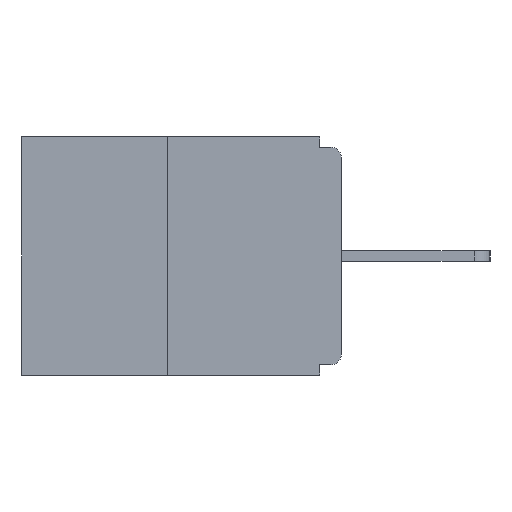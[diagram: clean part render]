
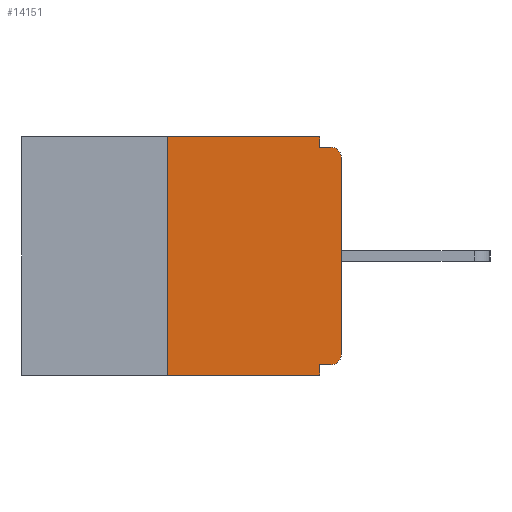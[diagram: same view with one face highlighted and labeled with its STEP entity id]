
A CAD part, left-side view. The second image highlights one B-rep face of the part: STEP entity #14151.
In plain terms, the highlighted planar face has unit normal (-1, 0, 0).
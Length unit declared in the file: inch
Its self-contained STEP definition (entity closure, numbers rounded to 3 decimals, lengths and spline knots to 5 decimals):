
#359 = VECTOR ( 'NONE', #7062, 39.37008 ) ;
#1234 = VECTOR ( 'NONE', #3320, 39.37008 ) ;
#2044 = EDGE_LOOP ( 'NONE', ( #13302, #2677, #19557, #24376, #18803, #3095, #15325, #21957, #6473, #6462 ) ) ;
#2048 = CARTESIAN_POINT ( 'NONE',  ( 0., 0.031, -0.015 ) ) ;
#2384 = VERTEX_POINT ( 'NONE', #6562 ) ;
#2677 = ORIENTED_EDGE ( 'NONE', *, *, #5023, .F. ) ;
#2897 = VERTEX_POINT ( 'NONE', #3703 ) ;
#2973 = AXIS2_PLACEMENT_3D ( 'NONE', #21497, #9699, #23426 ) ;
#3095 = ORIENTED_EDGE ( 'NONE', *, *, #13722, .T. ) ;
#3111 = AXIS2_PLACEMENT_3D ( 'NONE', #5977, #19871, #8029 ) ;
#3320 = DIRECTION ( 'NONE',  ( 0., -1., 0. ) ) ;
#3703 = CARTESIAN_POINT ( 'NONE',  ( 0., 0.015, -0.015 ) ) ;
#3969 = EDGE_CURVE ( 'NONE', #21044, #18635, #12084, .T. ) ;
#4061 = EDGE_CURVE ( 'NONE', #10122, #18208, #9629, .T. ) ;
#5023 = EDGE_CURVE ( 'NONE', #22409, #21044, #24588, .T. ) ;
#5128 = EDGE_CURVE ( 'NONE', #18635, #17248, #11715, .T. ) ;
#5430 = PLANE ( 'NONE',  #10316 ) ;
#5977 = CARTESIAN_POINT ( 'NONE',  ( 0., 0.015, -0.313 ) ) ;
#6462 = ORIENTED_EDGE ( 'NONE', *, *, #5128, .F. ) ;
#6473 = ORIENTED_EDGE ( 'NONE', *, *, #9023, .F. ) ;
#6562 = CARTESIAN_POINT ( 'NONE',  ( 0., 0., -0.313 ) ) ;
#6988 = CARTESIAN_POINT ( 'NONE',  ( 0., 0.031, -0.328 ) ) ;
#7062 = DIRECTION ( 'NONE',  ( 0., -1., 0. ) ) ;
#8029 = DIRECTION ( 'NONE',  ( 0., 0., -1. ) ) ;
#8273 = CARTESIAN_POINT ( 'NONE',  ( 0., 0., -0.328 ) ) ;
#9023 = EDGE_CURVE ( 'NONE', #17248, #2897, #16694, .T. ) ;
#9024 = LINE ( 'NONE', #8273, #18278 ) ;
#9426 = VERTEX_POINT ( 'NONE', #10624 ) ;
#9535 = DIRECTION ( 'NONE',  ( 0., 0., -1. ) ) ;
#9566 = LINE ( 'NONE', #11310, #23968 ) ;
#9629 = LINE ( 'NONE', #19759, #19477 ) ;
#9699 = DIRECTION ( 'NONE',  ( -1., 0., 0. ) ) ;
#9724 = CARTESIAN_POINT ( 'NONE',  ( 0., 0.031, -0.343 ) ) ;
#10122 = VERTEX_POINT ( 'NONE', #6988 ) ;
#10316 = AXIS2_PLACEMENT_3D ( 'NONE', #19342, #21327, #9535 ) ;
#10469 = DIRECTION ( 'NONE',  ( 0., 0., -1. ) ) ;
#10624 = CARTESIAN_POINT ( 'NONE',  ( 0., 0.015, -0.328 ) ) ;
#11213 = CIRCLE ( 'NONE', #2973, 0.015 ) ;
#11310 = CARTESIAN_POINT ( 'NONE',  ( 0., 0., 0. ) ) ;
#11676 = CARTESIAN_POINT ( 'NONE',  ( 0., 0.031, 0. ) ) ;
#11715 = LINE ( 'NONE', #11676, #21575 ) ;
#11869 = LINE ( 'NONE', #16972, #359 ) ;
#12084 = LINE ( 'NONE', #21326, #16700 ) ;
#12130 = CIRCLE ( 'NONE', #3111, 0.015 ) ;
#13293 = DIRECTION ( 'NONE',  ( 0., 0., 1. ) ) ;
#13302 = ORIENTED_EDGE ( 'NONE', *, *, #3969, .F. ) ;
#13722 = EDGE_CURVE ( 'NONE', #9426, #2384, #12130, .T. ) ;
#13802 = EDGE_CURVE ( 'NONE', #9426, #10122, #9024, .T. ) ;
#14151 = ADVANCED_FACE ( 'NONE', ( #19774 ), #5430, .F. ) ;
#15002 = DIRECTION ( 'NONE',  ( 0., 0., 1. ) ) ;
#15074 = VERTEX_POINT ( 'NONE', #18246 ) ;
#15325 = ORIENTED_EDGE ( 'NONE', *, *, #15701, .T. ) ;
#15506 = CARTESIAN_POINT ( 'NONE',  ( 0., 0.25, 0. ) ) ;
#15701 = EDGE_CURVE ( 'NONE', #2384, #15074, #9566, .T. ) ;
#16694 = LINE ( 'NONE', #17356, #1234 ) ;
#16700 = VECTOR ( 'NONE', #21345, 39.37008 ) ;
#16972 = CARTESIAN_POINT ( 'NONE',  ( 0., 0.46, -0.343 ) ) ;
#17248 = VERTEX_POINT ( 'NONE', #2048 ) ;
#17356 = CARTESIAN_POINT ( 'NONE',  ( 0., 0., -0.015 ) ) ;
#18208 = VERTEX_POINT ( 'NONE', #9724 ) ;
#18246 = CARTESIAN_POINT ( 'NONE',  ( 0., 0., -0.03 ) ) ;
#18278 = VECTOR ( 'NONE', #20121, 39.37008 ) ;
#18635 = VERTEX_POINT ( 'NONE', #18887 ) ;
#18803 = ORIENTED_EDGE ( 'NONE', *, *, #13802, .F. ) ;
#18887 = CARTESIAN_POINT ( 'NONE',  ( 0., 0.031, 0. ) ) ;
#19342 = CARTESIAN_POINT ( 'NONE',  ( 0., 0.46, 0. ) ) ;
#19477 = VECTOR ( 'NONE', #20001, 39.37008 ) ;
#19557 = ORIENTED_EDGE ( 'NONE', *, *, #22663, .T. ) ;
#19759 = CARTESIAN_POINT ( 'NONE',  ( 0., 0.031, -0.343 ) ) ;
#19774 = FACE_OUTER_BOUND ( 'NONE', #2044, .T. ) ;
#19871 = DIRECTION ( 'NONE',  ( -1., 0., 0. ) ) ;
#20001 = DIRECTION ( 'NONE',  ( 0., 0., -1. ) ) ;
#20121 = DIRECTION ( 'NONE',  ( 0., 1., 0. ) ) ;
#21044 = VERTEX_POINT ( 'NONE', #24639 ) ;
#21326 = CARTESIAN_POINT ( 'NONE',  ( 0., 0.46, 0. ) ) ;
#21327 = DIRECTION ( 'NONE',  ( 1., 0., 0. ) ) ;
#21345 = DIRECTION ( 'NONE',  ( 0., -1., 0. ) ) ;
#21497 = CARTESIAN_POINT ( 'NONE',  ( 0., 0.015, -0.03 ) ) ;
#21575 = VECTOR ( 'NONE', #10469, 39.37008 ) ;
#21957 = ORIENTED_EDGE ( 'NONE', *, *, #23481, .T. ) ;
#22044 = CARTESIAN_POINT ( 'NONE',  ( 0., 0.25, -0.343 ) ) ;
#22409 = VERTEX_POINT ( 'NONE', #22044 ) ;
#22663 = EDGE_CURVE ( 'NONE', #22409, #18208, #11869, .T. ) ;
#23426 = DIRECTION ( 'NONE',  ( 0., 0., -1. ) ) ;
#23481 = EDGE_CURVE ( 'NONE', #15074, #2897, #11213, .T. ) ;
#23968 = VECTOR ( 'NONE', #13293, 39.37008 ) ;
#23980 = VECTOR ( 'NONE', #15002, 39.37008 ) ;
#24376 = ORIENTED_EDGE ( 'NONE', *, *, #4061, .F. ) ;
#24588 = LINE ( 'NONE', #15506, #23980 ) ;
#24639 = CARTESIAN_POINT ( 'NONE',  ( 0., 0.25, 0. ) ) ;
